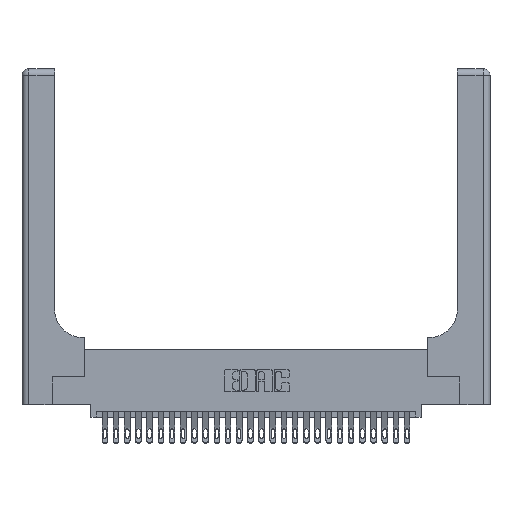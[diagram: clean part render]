
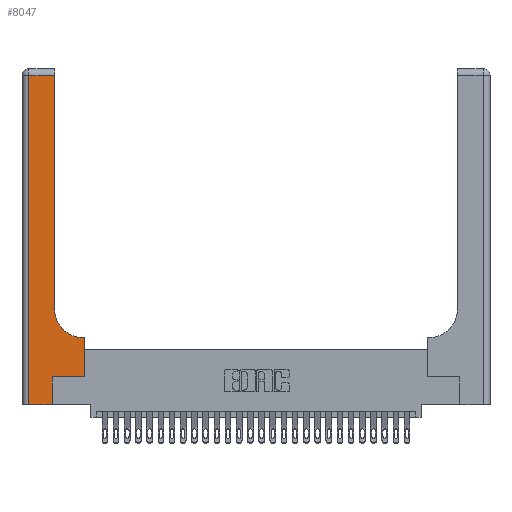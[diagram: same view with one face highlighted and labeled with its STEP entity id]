
A CAD part, top view. The second image highlights one B-rep face of the part: STEP entity #8047.
In plain terms, the highlighted planar face has unit normal (0, 0, 1).
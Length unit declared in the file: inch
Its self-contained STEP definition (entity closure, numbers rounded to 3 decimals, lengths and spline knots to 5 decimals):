
#175 = CARTESIAN_POINT ( 'NONE',  ( 0.5585, 0.25, 0.37 ) ) ;
#762 = CARTESIAN_POINT ( 'NONE',  ( 0.2915, 2.94, 0.37 ) ) ;
#1074 = ORIENTED_EDGE ( 'NONE', *, *, #13204, .T. ) ;
#1367 = DIRECTION ( 'NONE',  ( -1., 0., 0. ) ) ;
#1593 = DIRECTION ( 'NONE',  ( 1., 0., 0. ) ) ;
#1818 = CARTESIAN_POINT ( 'NONE',  ( 0.269, 0., 0.37 ) ) ;
#2289 = ORIENTED_EDGE ( 'NONE', *, *, #6141, .T. ) ;
#2366 = EDGE_CURVE ( 'NONE', #17367, #18673, #16471, .T. ) ;
#2615 = DIRECTION ( 'NONE',  ( 0., -1., 0. ) ) ;
#3028 = CARTESIAN_POINT ( 'NONE',  ( 0.06, 0., 0.37 ) ) ;
#3530 = VERTEX_POINT ( 'NONE', #762 ) ;
#3686 = CARTESIAN_POINT ( 'NONE',  ( 0., 3., 0.37 ) ) ;
#3703 = FACE_OUTER_BOUND ( 'NONE', #3873, .T. ) ;
#3800 = CARTESIAN_POINT ( 'NONE',  ( 0.06, 2.94, 0.37 ) ) ;
#3873 = EDGE_LOOP ( 'NONE', ( #27128, #19762, #18082, #12311, #2289, #4589, #16296, #1074, #25890 ) ) ;
#4384 = LINE ( 'NONE', #18020, #8991 ) ;
#4589 = ORIENTED_EDGE ( 'NONE', *, *, #20574, .T. ) ;
#5380 = CARTESIAN_POINT ( 'NONE',  ( 0.5585, 0.25, 0.37 ) ) ;
#6141 = EDGE_CURVE ( 'NONE', #18673, #18069, #20544, .T. ) ;
#7173 = CARTESIAN_POINT ( 'NONE',  ( 0.269, 0., 0.37 ) ) ;
#7439 = VECTOR ( 'NONE', #10138, 39.37008 ) ;
#7495 = CARTESIAN_POINT ( 'NONE',  ( 0.2915, 0.85, 0.37 ) ) ;
#7826 = EDGE_CURVE ( 'NONE', #7930, #8899, #11158, .T. ) ;
#7930 = VERTEX_POINT ( 'NONE', #12500 ) ;
#8047 = ADVANCED_FACE ( 'NONE', ( #3703 ), #26664, .F. ) ;
#8899 = VERTEX_POINT ( 'NONE', #7495 ) ;
#8991 = VECTOR ( 'NONE', #22615, 39.37008 ) ;
#9102 = DIRECTION ( 'NONE',  ( 1., 0., 0. ) ) ;
#9117 = EDGE_CURVE ( 'NONE', #3530, #25377, #26423, .T. ) ;
#9135 = DIRECTION ( 'NONE',  ( 0., 1., 0. ) ) ;
#9471 = LINE ( 'NONE', #13784, #16582 ) ;
#9701 = VECTOR ( 'NONE', #1593, 39.37008 ) ;
#10138 = DIRECTION ( 'NONE',  ( 0., 1., 0. ) ) ;
#10656 = CARTESIAN_POINT ( 'NONE',  ( 0.5585, 0.6, 0.37 ) ) ;
#11158 = CIRCLE ( 'NONE', #26566, 0.25 ) ;
#11901 = LINE ( 'NONE', #16125, #16918 ) ;
#12311 = ORIENTED_EDGE ( 'NONE', *, *, #2366, .T. ) ;
#12387 = VECTOR ( 'NONE', #9135, 39.37008 ) ;
#12500 = CARTESIAN_POINT ( 'NONE',  ( 0.5415, 0.6, 0.37 ) ) ;
#12790 = CARTESIAN_POINT ( 'NONE',  ( 0.269, 0.25, 0.37 ) ) ;
#13204 = EDGE_CURVE ( 'NONE', #19217, #7930, #4384, .T. ) ;
#13784 = CARTESIAN_POINT ( 'NONE',  ( 0.269, 0.25, 0.37 ) ) ;
#14755 = EDGE_CURVE ( 'NONE', #18338, #19217, #26709, .T. ) ;
#15429 = CARTESIAN_POINT ( 'NONE',  ( 0., 0., 0.37 ) ) ;
#15820 = CARTESIAN_POINT ( 'NONE',  ( 0.2915, 3., 0.37 ) ) ;
#16125 = CARTESIAN_POINT ( 'NONE',  ( 0.06, 3., 0.37 ) ) ;
#16296 = ORIENTED_EDGE ( 'NONE', *, *, #14755, .T. ) ;
#16471 = LINE ( 'NONE', #15429, #9701 ) ;
#16582 = VECTOR ( 'NONE', #9102, 39.37008 ) ;
#16918 = VECTOR ( 'NONE', #2615, 39.37008 ) ;
#17335 = VECTOR ( 'NONE', #24616, 39.37008 ) ;
#17367 = VERTEX_POINT ( 'NONE', #3028 ) ;
#17649 = CARTESIAN_POINT ( 'NONE',  ( 0., 2.94, 0.37 ) ) ;
#18020 = CARTESIAN_POINT ( 'NONE',  ( 0.2915, 0.6, 0.37 ) ) ;
#18069 = VERTEX_POINT ( 'NONE', #12790 ) ;
#18082 = ORIENTED_EDGE ( 'NONE', *, *, #27990, .T. ) ;
#18338 = VERTEX_POINT ( 'NONE', #175 ) ;
#18673 = VERTEX_POINT ( 'NONE', #7173 ) ;
#18706 = DIRECTION ( 'NONE',  ( 1., 0., 0. ) ) ;
#19217 = VERTEX_POINT ( 'NONE', #10656 ) ;
#19612 = DIRECTION ( 'NONE',  ( -1., 0., 0. ) ) ;
#19762 = ORIENTED_EDGE ( 'NONE', *, *, #9117, .T. ) ;
#19885 = LINE ( 'NONE', #15820, #12387 ) ;
#20368 = VECTOR ( 'NONE', #19612, 39.37008 ) ;
#20544 = LINE ( 'NONE', #1818, #17335 ) ;
#20574 = EDGE_CURVE ( 'NONE', #18069, #18338, #9471, .T. ) ;
#20713 = CARTESIAN_POINT ( 'NONE',  ( 0.5415, 0.85, 0.37 ) ) ;
#22615 = DIRECTION ( 'NONE',  ( -1., 0., 0. ) ) ;
#24616 = DIRECTION ( 'NONE',  ( 0., 1., 0. ) ) ;
#25377 = VERTEX_POINT ( 'NONE', #3800 ) ;
#25443 = EDGE_CURVE ( 'NONE', #8899, #3530, #19885, .T. ) ;
#25488 = DIRECTION ( 'NONE',  ( 0., 0., -1. ) ) ;
#25890 = ORIENTED_EDGE ( 'NONE', *, *, #7826, .T. ) ;
#26423 = LINE ( 'NONE', #17649, #20368 ) ;
#26566 = AXIS2_PLACEMENT_3D ( 'NONE', #20713, #25488, #18706 ) ;
#26664 = PLANE ( 'NONE',  #26970 ) ;
#26709 = LINE ( 'NONE', #5380, #7439 ) ;
#26970 = AXIS2_PLACEMENT_3D ( 'NONE', #3686, #28660, #1367 ) ;
#27128 = ORIENTED_EDGE ( 'NONE', *, *, #25443, .T. ) ;
#27990 = EDGE_CURVE ( 'NONE', #25377, #17367, #11901, .T. ) ;
#28660 = DIRECTION ( 'NONE',  ( 0., 0., -1. ) ) ;
